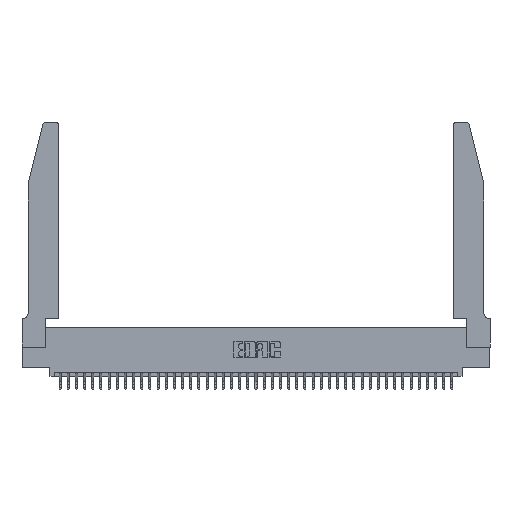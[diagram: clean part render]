
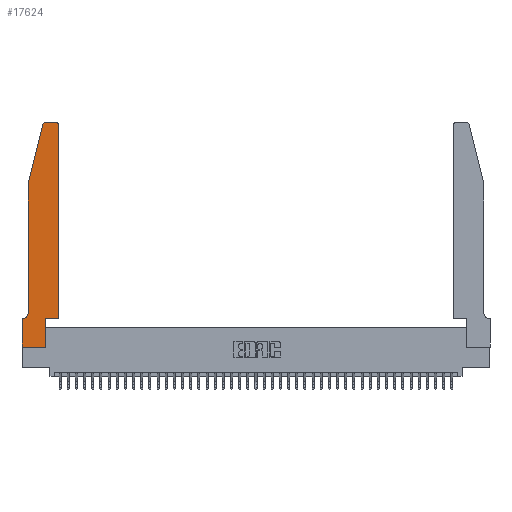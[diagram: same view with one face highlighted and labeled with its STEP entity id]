
A CAD part, top view. The second image highlights one B-rep face of the part: STEP entity #17624.
In plain terms, the highlighted planar face has unit normal (0, 0, 1).
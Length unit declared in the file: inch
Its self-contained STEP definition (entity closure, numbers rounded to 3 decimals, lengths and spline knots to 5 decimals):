
#16 = DIRECTION ( 'NONE',  ( 1., 0., 0. ) ) ;
#273 = DIRECTION ( 'NONE',  ( 1., 0., 0. ) ) ;
#448 = ORIENTED_EDGE ( 'NONE', *, *, #38592, .T. ) ;
#1646 = ORIENTED_EDGE ( 'NONE', *, *, #19721, .T. ) ;
#1825 = VERTEX_POINT ( 'NONE', #32491 ) ;
#1905 = LINE ( 'NONE', #29678, #19517 ) ;
#2383 = ORIENTED_EDGE ( 'NONE', *, *, #13363, .T. ) ;
#3314 = DIRECTION ( 'NONE',  ( 1., 0., 0. ) ) ;
#3321 = VERTEX_POINT ( 'NONE', #8219 ) ;
#3346 = ORIENTED_EDGE ( 'NONE', *, *, #16203, .T. ) ;
#3526 = CARTESIAN_POINT ( 'NONE',  ( 0.0055, 0.42, 0.37 ) ) ;
#4356 = DIRECTION ( 'NONE',  ( 0., -1., 0. ) ) ;
#5089 = LINE ( 'NONE', #9203, #30328 ) ;
#6196 = EDGE_CURVE ( 'NONE', #32650, #38179, #9355, .T. ) ;
#6822 = CARTESIAN_POINT ( 'NONE',  ( 0.0755, 2., 0.37 ) ) ;
#6852 = DIRECTION ( 'NONE',  ( -1., 0., 0. ) ) ;
#8219 = CARTESIAN_POINT ( 'NONE',  ( 0.25487, 2.72718, 0.37 ) ) ;
#8220 = DIRECTION ( 'NONE',  ( 0., 0., 1. ) ) ;
#8231 = VECTOR ( 'NONE', #15333, 39.37008 ) ;
#8667 = VERTEX_POINT ( 'NONE', #27612 ) ;
#8977 = CARTESIAN_POINT ( 'NONE',  ( 0.4505, 2.72, 0.37 ) ) ;
#9203 = CARTESIAN_POINT ( 'NONE',  ( 0.2605, 2.75, 0.37 ) ) ;
#9355 = CIRCLE ( 'NONE', #31580, 0.03 ) ;
#10375 = CARTESIAN_POINT ( 'NONE',  ( 0.2865, 0., 0.37 ) ) ;
#11442 = LINE ( 'NONE', #21358, #27884 ) ;
#12377 = CARTESIAN_POINT ( 'NONE',  ( 0., 0., 0.37 ) ) ;
#12471 = VERTEX_POINT ( 'NONE', #6822 ) ;
#12780 = VERTEX_POINT ( 'NONE', #25089 ) ;
#13083 = VECTOR ( 'NONE', #21348, 39.37008 ) ;
#13363 = EDGE_CURVE ( 'NONE', #27307, #32650, #30525, .T. ) ;
#13729 = VERTEX_POINT ( 'NONE', #10375 ) ;
#13747 = CARTESIAN_POINT ( 'NONE',  ( 0.0755, 0.35, 0.37 ) ) ;
#14529 = CIRCLE ( 'NONE', #36022, 0.03 ) ;
#14643 = ORIENTED_EDGE ( 'NONE', *, *, #34828, .T. ) ;
#15249 = LINE ( 'NONE', #16309, #29600 ) ;
#15273 = CARTESIAN_POINT ( 'NONE',  ( 0.4505, 0.35, 0.37 ) ) ;
#15289 = ORIENTED_EDGE ( 'NONE', *, *, #31182, .T. ) ;
#15333 = DIRECTION ( 'NONE',  ( 0., 1., 0. ) ) ;
#15669 = ORIENTED_EDGE ( 'NONE', *, *, #31546, .T. ) ;
#16203 = EDGE_CURVE ( 'NONE', #20529, #13729, #1905, .T. ) ;
#16309 = CARTESIAN_POINT ( 'NONE',  ( 0.0755, 2., 0.37 ) ) ;
#17624 = ADVANCED_FACE ( 'NONE', ( #30735 ), #39745, .T. ) ;
#18492 = CARTESIAN_POINT ( 'NONE',  ( 0.0755, 0.42, 0.37 ) ) ;
#19171 = DIRECTION ( 'NONE',  ( -1., 0., 0. ) ) ;
#19232 = VECTOR ( 'NONE', #4356, 39.37008 ) ;
#19517 = VECTOR ( 'NONE', #3314, 39.37008 ) ;
#19721 = EDGE_CURVE ( 'NONE', #13729, #34204, #36511, .T. ) ;
#19873 = DIRECTION ( 'NONE',  ( 0., 0., 1. ) ) ;
#20129 = DIRECTION ( 'NONE',  ( 0., 0., 1. ) ) ;
#20271 = LINE ( 'NONE', #33849, #19232 ) ;
#20529 = VERTEX_POINT ( 'NONE', #12377 ) ;
#20875 = AXIS2_PLACEMENT_3D ( 'NONE', #3526, #26594, #6852 ) ;
#21123 = ORIENTED_EDGE ( 'NONE', *, *, #39615, .T. ) ;
#21348 = DIRECTION ( 'NONE',  ( 0., 1., 0. ) ) ;
#21358 = CARTESIAN_POINT ( 'NONE',  ( 0.0755, 2., 0.37 ) ) ;
#21665 = CARTESIAN_POINT ( 'NONE',  ( 0.2865, 0.35, 0.37 ) ) ;
#24313 = EDGE_CURVE ( 'NONE', #1825, #12780, #26386, .T. ) ;
#24648 = DIRECTION ( 'NONE',  ( 0., -1., 0. ) ) ;
#25089 = CARTESIAN_POINT ( 'NONE',  ( 0., 0.35, 0.37 ) ) ;
#26057 = ORIENTED_EDGE ( 'NONE', *, *, #41298, .T. ) ;
#26386 = LINE ( 'NONE', #13747, #34080 ) ;
#26413 = VERTEX_POINT ( 'NONE', #18492 ) ;
#26594 = DIRECTION ( 'NONE',  ( 0., 0., -1. ) ) ;
#27307 = VERTEX_POINT ( 'NONE', #30807 ) ;
#27612 = CARTESIAN_POINT ( 'NONE',  ( 0.284, 2.75, 0.37 ) ) ;
#27884 = VECTOR ( 'NONE', #24648, 39.37008 ) ;
#27949 = CARTESIAN_POINT ( 'NONE',  ( 0.4205, 2.72, 0.37 ) ) ;
#28501 = ORIENTED_EDGE ( 'NONE', *, *, #24313, .T. ) ;
#28557 = CARTESIAN_POINT ( 'NONE',  ( 0.4205, 2.75, 0.37 ) ) ;
#28840 = ORIENTED_EDGE ( 'NONE', *, *, #6196, .T. ) ;
#29600 = VECTOR ( 'NONE', #42490, 39.37008 ) ;
#29678 = CARTESIAN_POINT ( 'NONE',  ( 0., 0., 0.37 ) ) ;
#29865 = CARTESIAN_POINT ( 'NONE',  ( 0., 0.35, 0.37 ) ) ;
#30328 = VECTOR ( 'NONE', #19171, 39.37008 ) ;
#30525 = LINE ( 'NONE', #37635, #13083 ) ;
#30735 = FACE_OUTER_BOUND ( 'NONE', #36875, .T. ) ;
#30807 = CARTESIAN_POINT ( 'NONE',  ( 0.4505, 0.35, 0.37 ) ) ;
#31182 = EDGE_CURVE ( 'NONE', #12471, #26413, #11442, .T. ) ;
#31207 = DIRECTION ( 'NONE',  ( 1., 0., 0. ) ) ;
#31546 = EDGE_CURVE ( 'NONE', #8667, #3321, #14529, .T. ) ;
#31577 = DIRECTION ( 'NONE',  ( 1., 0., 0. ) ) ;
#31580 = AXIS2_PLACEMENT_3D ( 'NONE', #27949, #8220, #31207 ) ;
#31868 = EDGE_CURVE ( 'NONE', #34204, #27307, #37033, .T. ) ;
#32087 = CARTESIAN_POINT ( 'NONE',  ( 0.2865, 0.35, 0.37 ) ) ;
#32491 = CARTESIAN_POINT ( 'NONE',  ( 0.0055, 0.35, 0.37 ) ) ;
#32650 = VERTEX_POINT ( 'NONE', #8977 ) ;
#33849 = CARTESIAN_POINT ( 'NONE',  ( 0., 0., 0.37 ) ) ;
#34080 = VECTOR ( 'NONE', #39967, 39.37008 ) ;
#34204 = VERTEX_POINT ( 'NONE', #32087 ) ;
#34828 = EDGE_CURVE ( 'NONE', #3321, #12471, #15249, .T. ) ;
#34904 = AXIS2_PLACEMENT_3D ( 'NONE', #29865, #20129, #273 ) ;
#36000 = VECTOR ( 'NONE', #31577, 39.37008 ) ;
#36022 = AXIS2_PLACEMENT_3D ( 'NONE', #39494, #19873, #16 ) ;
#36511 = LINE ( 'NONE', #21665, #8231 ) ;
#36875 = EDGE_LOOP ( 'NONE', ( #26057, #15669, #14643, #15289, #21123, #28501, #448, #3346, #1646, #39941, #2383, #28840 ) ) ;
#37033 = LINE ( 'NONE', #15273, #36000 ) ;
#37635 = CARTESIAN_POINT ( 'NONE',  ( 0.4505, 0.35, 0.37 ) ) ;
#38179 = VERTEX_POINT ( 'NONE', #28557 ) ;
#38592 = EDGE_CURVE ( 'NONE', #12780, #20529, #20271, .T. ) ;
#39494 = CARTESIAN_POINT ( 'NONE',  ( 0.284, 2.72, 0.37 ) ) ;
#39615 = EDGE_CURVE ( 'NONE', #26413, #1825, #42175, .T. ) ;
#39745 = PLANE ( 'NONE',  #34904 ) ;
#39941 = ORIENTED_EDGE ( 'NONE', *, *, #31868, .T. ) ;
#39967 = DIRECTION ( 'NONE',  ( -1., 0., 0. ) ) ;
#41298 = EDGE_CURVE ( 'NONE', #38179, #8667, #5089, .T. ) ;
#42175 = CIRCLE ( 'NONE', #20875, 0.07 ) ;
#42490 = DIRECTION ( 'NONE',  ( -0.239, -0.971, 0. ) ) ;
